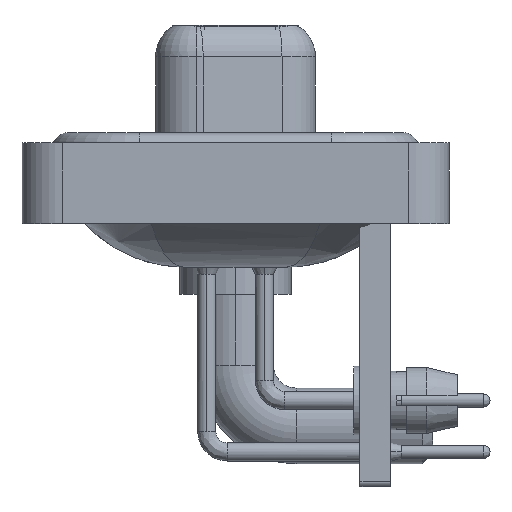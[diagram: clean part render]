
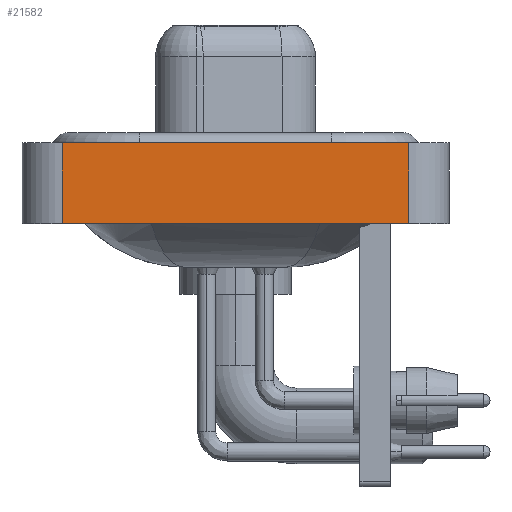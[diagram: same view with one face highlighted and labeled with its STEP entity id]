
A CAD part, left-side view. The second image highlights one B-rep face of the part: STEP entity #21582.
In plain terms, the highlighted planar face has unit normal (-1, 0, 0).
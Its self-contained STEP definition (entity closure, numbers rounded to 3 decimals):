
#515 = CARTESIAN_POINT ( 'NONE',  ( -7.3, 8.55, 0.4 ) ) ;
#757 = CARTESIAN_POINT ( 'NONE',  ( -7.3, -8.55, -3.6 ) ) ;
#1441 = DIRECTION ( 'NONE',  ( 0., 0., 1. ) ) ;
#2256 = VECTOR ( 'NONE', #3530, 1000. ) ;
#2565 = CARTESIAN_POINT ( 'NONE',  ( -7.3, 8.55, -3.6 ) ) ;
#3117 = EDGE_LOOP ( 'NONE', ( #17356, #14500, #17361, #3262 ) ) ;
#3221 = AXIS2_PLACEMENT_3D ( 'NONE', #16131, #23913, #12484 ) ;
#3262 = ORIENTED_EDGE ( 'NONE', *, *, #13493, .T. ) ;
#3349 = CARTESIAN_POINT ( 'NONE',  ( -7.3, -8.55, -3.6 ) ) ;
#3530 = DIRECTION ( 'NONE',  ( 0., -1., 0. ) ) ;
#4125 = CARTESIAN_POINT ( 'NONE',  ( -7.3, -8.55, 0.4 ) ) ;
#4878 = EDGE_CURVE ( 'NONE', #19221, #19934, #19795, .T. ) ;
#5278 = EDGE_CURVE ( 'NONE', #19934, #22974, #7309, .T. ) ;
#6076 = VECTOR ( 'NONE', #1441, 1000. ) ;
#7078 = VECTOR ( 'NONE', #12260, 1000. ) ;
#7189 = LINE ( 'NONE', #20386, #8748 ) ;
#7309 = LINE ( 'NONE', #18245, #2256 ) ;
#8748 = VECTOR ( 'NONE', #22389, 1000. ) ;
#9031 = EDGE_CURVE ( 'NONE', #13339, #22974, #14908, .T. ) ;
#11660 = CARTESIAN_POINT ( 'NONE',  ( -7.3, 8.55, -3.6 ) ) ;
#12260 = DIRECTION ( 'NONE',  ( 0., 0., 1. ) ) ;
#12484 = DIRECTION ( 'NONE',  ( 0., 0., 1. ) ) ;
#13339 = VERTEX_POINT ( 'NONE', #757 ) ;
#13493 = EDGE_CURVE ( 'NONE', #19221, #13339, #7189, .T. ) ;
#14237 = FACE_OUTER_BOUND ( 'NONE', #3117, .T. ) ;
#14500 = ORIENTED_EDGE ( 'NONE', *, *, #5278, .F. ) ;
#14908 = LINE ( 'NONE', #3349, #6076 ) ;
#16131 = CARTESIAN_POINT ( 'NONE',  ( -7.3, -8.55, -3.6 ) ) ;
#17356 = ORIENTED_EDGE ( 'NONE', *, *, #9031, .T. ) ;
#17361 = ORIENTED_EDGE ( 'NONE', *, *, #4878, .F. ) ;
#18245 = CARTESIAN_POINT ( 'NONE',  ( -7.3, -8.55, 0.4 ) ) ;
#19221 = VERTEX_POINT ( 'NONE', #11660 ) ;
#19795 = LINE ( 'NONE', #2565, #7078 ) ;
#19934 = VERTEX_POINT ( 'NONE', #515 ) ;
#20386 = CARTESIAN_POINT ( 'NONE',  ( -7.3, -8.55, -3.6 ) ) ;
#21582 = ADVANCED_FACE ( 'NONE', ( #14237 ), #21775, .T. ) ;
#21775 = PLANE ( 'NONE',  #3221 ) ;
#22389 = DIRECTION ( 'NONE',  ( 0., -1., 0. ) ) ;
#22974 = VERTEX_POINT ( 'NONE', #4125 ) ;
#23913 = DIRECTION ( 'NONE',  ( -1., 0., 0. ) ) ;
